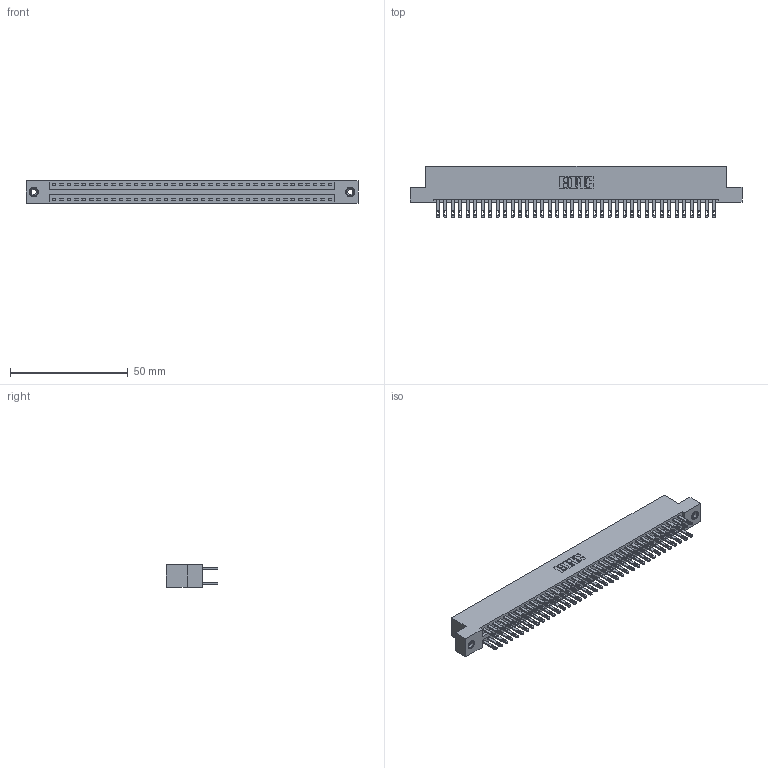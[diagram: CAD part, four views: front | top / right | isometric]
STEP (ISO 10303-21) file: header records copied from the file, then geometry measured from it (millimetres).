
FILE_DESCRIPTION (( 'STEP AP203' ), '1' );
FILE_NAME ('896-076-500-208.STEP', '2021-07-28T01:43:05', ( '' ), ( '' ), 'SwSTEP 2.0', 'SolidWorks 2020', '' );
FILE_SCHEMA (( 'CONFIG_CONTROL_DESIGN' ));
Length unit declared in the file: inch
Products named in the file (4): 345-250-001_345-250-003-102; 846 Part_Flush Mounting Lugs - 0.156 Dia-TI; 896-076-500-208; 345-292-001_345-293-100
Assembly tree (79 placements, depth 2):
  896-076-500-208
    846 Part_Flush Mounting Lugs - 0.156 Dia-TI
    345-292-001_345-293-100  x76
    345-250-001_345-250-003-102  x2
Bounding box: 141.22 x 21.84 x 9.4 mm (x, y, z)
Volume: 13965.8 mm3; surface area: 19949.5 mm2
Topology: 79 solids, 79 shells, 3830 faces, 11637 edges, 7750 vertices
Faces by surface type: plane 2312, cylinder 1502, cone 12, torus 4
Entity records: 26454 total; most frequent: CARTESIAN_POINT 4347, ORIENTED_EDGE 4274, DIRECTION 3911, EDGE_CURVE 2137, VECTOR 1829, LINE 1829, VERTEX_POINT 1420, AXIS2_PLACEMENT_3D 1041
